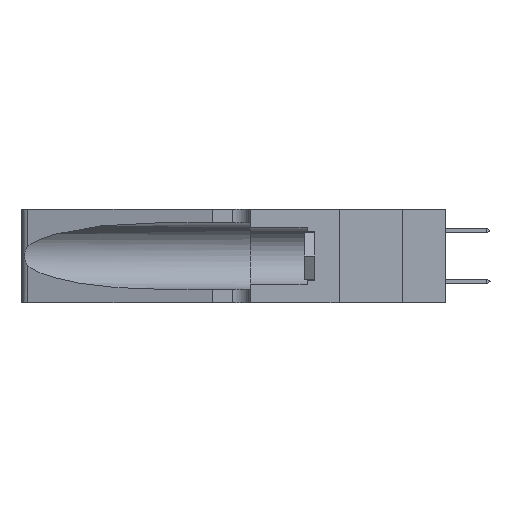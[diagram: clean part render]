
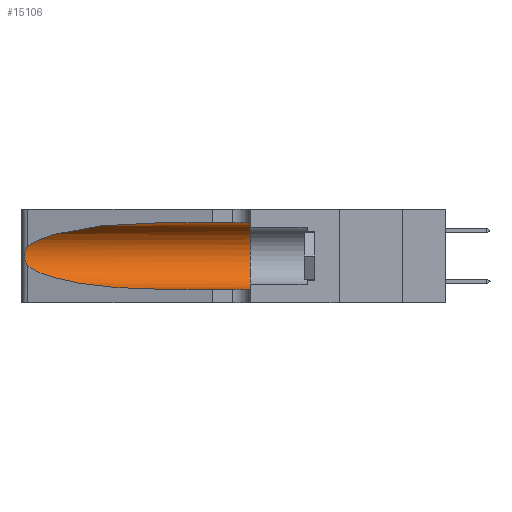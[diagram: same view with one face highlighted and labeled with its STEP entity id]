
A CAD part, left-side view. The second image highlights one B-rep face of the part: STEP entity #15106.
In plain terms, the highlighted cylindrical face has radius 3.308 mm (diameter 6.617 mm), a partial arc.
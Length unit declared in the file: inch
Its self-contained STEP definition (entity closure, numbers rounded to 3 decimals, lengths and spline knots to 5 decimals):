
#706 = EDGE_LOOP ( 'NONE', ( #3882, #7452, #21391, #17147, #21173, #28061 ) ) ;
#1794 =( BOUNDED_CURVE ( )  B_SPLINE_CURVE ( 3, ( #17559, #6133, #8472, #8668 ),
 .UNSPECIFIED., .F., .F. ) 
 B_SPLINE_CURVE_WITH_KNOTS ( ( 4, 4 ),
 ( 1.5708, 2.84003 ),
 .UNSPECIFIED. ) 
 CURVE ( )  GEOMETRIC_REPRESENTATION_ITEM ( )  RATIONAL_B_SPLINE_CURVE ( ( 1., 0.87, 0.87, 1. ) ) 
 REPRESENTATION_ITEM ( '' )  );
#2693 = AXIS2_PLACEMENT_3D ( 'NONE', #28388, #19150, #17004 ) ;
#3002 = CARTESIAN_POINT ( 'NONE',  ( 0.25487, 1.22718, 0.22369 ) ) ;
#3279 = VERTEX_POINT ( 'NONE', #20690 ) ;
#3495 = CARTESIAN_POINT ( 'NONE',  ( 0.18966, 0.96281, 0.05475 ) ) ;
#3882 = ORIENTED_EDGE ( 'NONE', *, *, #18364, .T. ) ;
#4478 = CARTESIAN_POINT ( 'NONE',  ( 0.1305, 0.35, 0.31525 ) ) ;
#5469 = CARTESIAN_POINT ( 'NONE',  ( 0.1305, 0.35, 0.185 ) ) ;
#5676 = CARTESIAN_POINT ( 'NONE',  ( 0.1305, 0.72297, 0.05475 ) ) ;
#5683 = DIRECTION ( 'NONE',  ( 0., 1., 0. ) ) ;
#6133 = CARTESIAN_POINT ( 'NONE',  ( 0.18966, 0.96281, 0.31525 ) ) ;
#6737 = VERTEX_POINT ( 'NONE', #4478 ) ;
#7003 = EDGE_CURVE ( 'NONE', #24716, #12817, #18809, .T. ) ;
#7248 = DIRECTION ( 'NONE',  ( 0., -1., 0. ) ) ;
#7452 = ORIENTED_EDGE ( 'NONE', *, *, #14029, .T. ) ;
#8270 = CARTESIAN_POINT ( 'NONE',  ( 0.25555, 1.22993, 0.14849 ) ) ;
#8289 = CARTESIAN_POINT ( 'NONE',  ( 0.2373, 1.15595, 0.08982 ) ) ;
#8472 = CARTESIAN_POINT ( 'NONE',  ( 0.2373, 1.15595, 0.28018 ) ) ;
#8668 = CARTESIAN_POINT ( 'NONE',  ( 0.25487, 1.22718, 0.22369 ) ) ;
#9462 = CARTESIAN_POINT ( 'NONE',  ( 0.1305, 1.61858, 0.31525 ) ) ;
#10506 = VERTEX_POINT ( 'NONE', #23988 ) ;
#10625 = CARTESIAN_POINT ( 'NONE',  ( 0.1305, 0.72297, 0.05475 ) ) ;
#10738 = CARTESIAN_POINT ( 'NONE',  ( 0.25487, 1.22718, 0.14631 ) ) ;
#10747 = CARTESIAN_POINT ( 'NONE',  ( 0.25639, 1.23186, 0.15144 ) ) ;
#11836 = CARTESIAN_POINT ( 'NONE',  ( 0.26075, 1.23896, 0.178 ) ) ;
#12817 = VERTEX_POINT ( 'NONE', #21513 ) ;
#13838 = DIRECTION ( 'NONE',  ( 0., -1., 0. ) ) ;
#14029 = EDGE_CURVE ( 'NONE', #3279, #10506, #25646, .T. ) ;
#14078 = CYLINDRICAL_SURFACE ( 'NONE', #2693, 0.13025 ) ;
#15106 = ADVANCED_FACE ( 'NONE', ( #15879 ), #14078, .F. ) ;
#15879 = FACE_OUTER_BOUND ( 'NONE', #706, .T. ) ;
#17004 = DIRECTION ( 'NONE',  ( 0., 0., -1. ) ) ;
#17021 =( BOUNDED_CURVE ( )  B_SPLINE_CURVE ( 3, ( #10738, #8289, #3495, #10625 ),
 .UNSPECIFIED., .F., .T. ) 
 B_SPLINE_CURVE_WITH_KNOTS ( ( 4, 4 ),
 ( 3.44316, 4.71239 ),
 .UNSPECIFIED. ) 
 CURVE ( )  GEOMETRIC_REPRESENTATION_ITEM ( )  RATIONAL_B_SPLINE_CURVE ( ( 1., 0.87, 0.87, 1. ) ) 
 REPRESENTATION_ITEM ( '' )  );
#17147 = ORIENTED_EDGE ( 'NONE', *, *, #7003, .T. ) ;
#17420 = CARTESIAN_POINT ( 'NONE',  ( 0.25555, 1.22994, 0.2215 ) ) ;
#17559 = CARTESIAN_POINT ( 'NONE',  ( 0.1305, 0.72297, 0.31525 ) ) ;
#18364 = EDGE_CURVE ( 'NONE', #27801, #3279, #1794, .T. ) ;
#18809 = LINE ( 'NONE', #20252, #23211 ) ;
#19150 = DIRECTION ( 'NONE',  ( 0., -1., 0. ) ) ;
#19600 = EDGE_CURVE ( 'NONE', #10506, #24716, #17021, .T. ) ;
#19826 = CARTESIAN_POINT ( 'NONE',  ( 0.26018, 1.23835, 0.19895 ) ) ;
#20252 = CARTESIAN_POINT ( 'NONE',  ( 0.1305, 1.61858, 0.05475 ) ) ;
#20690 = CARTESIAN_POINT ( 'NONE',  ( 0.25487, 1.22718, 0.22369 ) ) ;
#21173 = ORIENTED_EDGE ( 'NONE', *, *, #21357, .F. ) ;
#21357 = EDGE_CURVE ( 'NONE', #6737, #12817, #29923, .T. ) ;
#21391 = ORIENTED_EDGE ( 'NONE', *, *, #19600, .T. ) ;
#21513 = CARTESIAN_POINT ( 'NONE',  ( 0.1305, 0.35, 0.05475 ) ) ;
#21791 = CARTESIAN_POINT ( 'NONE',  ( 0.25787, 1.23484, 0.2124 ) ) ;
#22808 = VECTOR ( 'NONE', #7248, 39.37008 ) ;
#22970 = CARTESIAN_POINT ( 'NONE',  ( 0.25789, 1.23486, 0.15765 ) ) ;
#23029 = CARTESIAN_POINT ( 'NONE',  ( 0.25854, 1.2359, 0.20912 ) ) ;
#23211 = VECTOR ( 'NONE', #13838, 39.37008 ) ;
#23988 = CARTESIAN_POINT ( 'NONE',  ( 0.25487, 1.22718, 0.14631 ) ) ;
#24388 = EDGE_CURVE ( 'NONE', #27801, #6737, #28297, .T. ) ;
#24716 = VERTEX_POINT ( 'NONE', #5676 ) ;
#25268 = CARTESIAN_POINT ( 'NONE',  ( 0.26017, 1.23833, 0.17102 ) ) ;
#25590 = CARTESIAN_POINT ( 'NONE',  ( 0.1305, 0.72297, 0.31525 ) ) ;
#25646 = B_SPLINE_CURVE_WITH_KNOTS ( 'NONE', 3,
 ( #3002, #17420, #26934, #21791, #23029, #19826, #27619, #11836, #25268, #26910, #22970, #10747, #8270, #29610 ),
 .UNSPECIFIED., .F., .F.,
 ( 4, 2, 2, 2, 2, 2, 4 ),
 ( 0., 0.00027, 0.00053, 0.00107, 0.0016, 0.00187, 0.00214 ),
 .UNSPECIFIED. ) ;
#26910 = CARTESIAN_POINT ( 'NONE',  ( 0.25856, 1.23593, 0.16098 ) ) ;
#26934 = CARTESIAN_POINT ( 'NONE',  ( 0.25639, 1.23184, 0.21858 ) ) ;
#27451 = AXIS2_PLACEMENT_3D ( 'NONE', #5469, #5683, #29004 ) ;
#27619 = CARTESIAN_POINT ( 'NONE',  ( 0.26075, 1.23896, 0.19203 ) ) ;
#27801 = VERTEX_POINT ( 'NONE', #25590 ) ;
#28061 = ORIENTED_EDGE ( 'NONE', *, *, #24388, .F. ) ;
#28297 = LINE ( 'NONE', #9462, #22808 ) ;
#28388 = CARTESIAN_POINT ( 'NONE',  ( 0.1305, 1.61858, 0.185 ) ) ;
#29004 = DIRECTION ( 'NONE',  ( 0., 0., 1. ) ) ;
#29610 = CARTESIAN_POINT ( 'NONE',  ( 0.25487, 1.22718, 0.14631 ) ) ;
#29923 = CIRCLE ( 'NONE', #27451, 0.13025 ) ;
